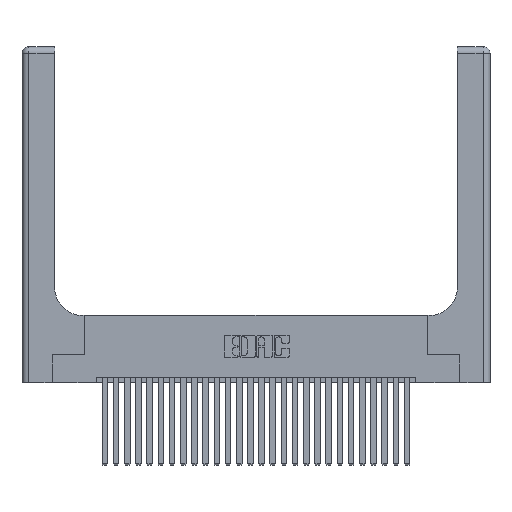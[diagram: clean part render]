
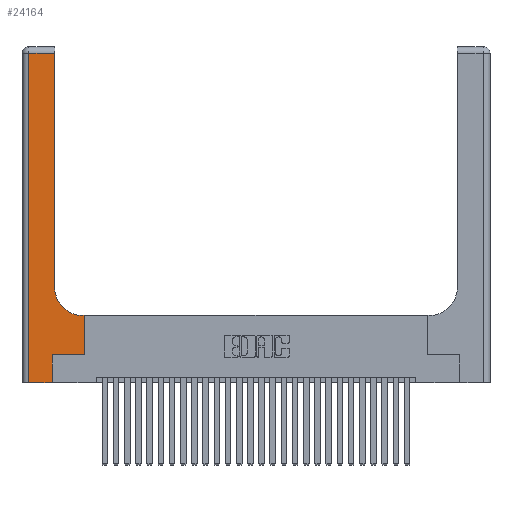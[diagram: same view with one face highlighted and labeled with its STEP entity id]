
A CAD part, top view. The second image highlights one B-rep face of the part: STEP entity #24164.
In plain terms, the highlighted planar face has unit normal (0, 0, 1).
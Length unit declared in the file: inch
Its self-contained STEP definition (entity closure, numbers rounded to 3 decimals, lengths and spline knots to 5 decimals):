
#298 = VERTEX_POINT ( 'NONE', #4008 ) ;
#327 = LINE ( 'NONE', #25647, #7044 ) ;
#1005 = VECTOR ( 'NONE', #8817, 39.37008 ) ;
#1125 = DIRECTION ( 'NONE',  ( 0., 0., -1. ) ) ;
#1407 = EDGE_CURVE ( 'NONE', #298, #4816, #18150, .T. ) ;
#1796 = ORIENTED_EDGE ( 'NONE', *, *, #18109, .T. ) ;
#2268 = EDGE_CURVE ( 'NONE', #15650, #21224, #3063, .T. ) ;
#2688 = VERTEX_POINT ( 'NONE', #15020 ) ;
#3062 = ORIENTED_EDGE ( 'NONE', *, *, #1407, .T. ) ;
#3063 = CIRCLE ( 'NONE', #17693, 0.25 ) ;
#3079 = DIRECTION ( 'NONE',  ( 1., 0., 0. ) ) ;
#3293 = CARTESIAN_POINT ( 'NONE',  ( 0.2915, 0.6, 0.37 ) ) ;
#3339 = CARTESIAN_POINT ( 'NONE',  ( 0.5585, 0.25, 0.37 ) ) ;
#3639 = CARTESIAN_POINT ( 'NONE',  ( 0.2915, 0.85, 0.37 ) ) ;
#4008 = CARTESIAN_POINT ( 'NONE',  ( 0.5585, 0.25, 0.37 ) ) ;
#4056 = CARTESIAN_POINT ( 'NONE',  ( 0.06, 3., 0.37 ) ) ;
#4513 = CARTESIAN_POINT ( 'NONE',  ( 0.5415, 0.85, 0.37 ) ) ;
#4816 = VERTEX_POINT ( 'NONE', #13047 ) ;
#5279 = LINE ( 'NONE', #3293, #16467 ) ;
#6472 = FACE_OUTER_BOUND ( 'NONE', #11373, .T. ) ;
#6727 = DIRECTION ( 'NONE',  ( 1., 0., 0. ) ) ;
#7044 = VECTOR ( 'NONE', #27852, 39.37008 ) ;
#7307 = LINE ( 'NONE', #4056, #13261 ) ;
#7729 = LINE ( 'NONE', #27632, #24783 ) ;
#7750 = CARTESIAN_POINT ( 'NONE',  ( 0.5415, 0.6, 0.37 ) ) ;
#7824 = DIRECTION ( 'NONE',  ( 0., 1., 0. ) ) ;
#8817 = DIRECTION ( 'NONE',  ( -1., 0., 0. ) ) ;
#9184 = EDGE_CURVE ( 'NONE', #19951, #298, #327, .T. ) ;
#9805 = VERTEX_POINT ( 'NONE', #23495 ) ;
#10004 = VECTOR ( 'NONE', #10326, 39.37008 ) ;
#10326 = DIRECTION ( 'NONE',  ( 0., 1., 0. ) ) ;
#10386 = ORIENTED_EDGE ( 'NONE', *, *, #2268, .T. ) ;
#10901 = EDGE_CURVE ( 'NONE', #9805, #2688, #12663, .T. ) ;
#11137 = CARTESIAN_POINT ( 'NONE',  ( 0.06, 2.94, 0.37 ) ) ;
#11282 = DIRECTION ( 'NONE',  ( 0., 1., 0. ) ) ;
#11373 = EDGE_LOOP ( 'NONE', ( #27351, #1796, #19914, #27807, #18780, #25518, #3062, #13620, #10386 ) ) ;
#11813 = DIRECTION ( 'NONE',  ( -1., 0., 0. ) ) ;
#12663 = LINE ( 'NONE', #20819, #23082 ) ;
#12683 = CARTESIAN_POINT ( 'NONE',  ( 0.2915, 2.94, 0.37 ) ) ;
#13047 = CARTESIAN_POINT ( 'NONE',  ( 0.5585, 0.6, 0.37 ) ) ;
#13261 = VECTOR ( 'NONE', #19632, 39.37008 ) ;
#13620 = ORIENTED_EDGE ( 'NONE', *, *, #27261, .T. ) ;
#15020 = CARTESIAN_POINT ( 'NONE',  ( 0.269, 0., 0.37 ) ) ;
#15332 = VERTEX_POINT ( 'NONE', #11137 ) ;
#15650 = VERTEX_POINT ( 'NONE', #7750 ) ;
#16467 = VECTOR ( 'NONE', #11813, 39.37008 ) ;
#16825 = DIRECTION ( 'NONE',  ( -1., 0., 0. ) ) ;
#17640 = EDGE_CURVE ( 'NONE', #21224, #24825, #7729, .T. ) ;
#17693 = AXIS2_PLACEMENT_3D ( 'NONE', #4513, #20079, #6727 ) ;
#17885 = CARTESIAN_POINT ( 'NONE',  ( 0.269, 0.25, 0.37 ) ) ;
#18109 = EDGE_CURVE ( 'NONE', #24825, #15332, #19564, .T. ) ;
#18150 = LINE ( 'NONE', #3339, #24010 ) ;
#18780 = ORIENTED_EDGE ( 'NONE', *, *, #23553, .T. ) ;
#19564 = LINE ( 'NONE', #19906, #1005 ) ;
#19632 = DIRECTION ( 'NONE',  ( 0., -1., 0. ) ) ;
#19906 = CARTESIAN_POINT ( 'NONE',  ( 0., 2.94, 0.37 ) ) ;
#19914 = ORIENTED_EDGE ( 'NONE', *, *, #28106, .T. ) ;
#19951 = VERTEX_POINT ( 'NONE', #17885 ) ;
#20079 = DIRECTION ( 'NONE',  ( 0., 0., -1. ) ) ;
#20819 = CARTESIAN_POINT ( 'NONE',  ( 0., 0., 0.37 ) ) ;
#21224 = VERTEX_POINT ( 'NONE', #3639 ) ;
#21373 = CARTESIAN_POINT ( 'NONE',  ( 0.269, 0., 0.37 ) ) ;
#21768 = AXIS2_PLACEMENT_3D ( 'NONE', #27799, #1125, #16825 ) ;
#21804 = LINE ( 'NONE', #21373, #10004 ) ;
#23082 = VECTOR ( 'NONE', #3079, 39.37008 ) ;
#23378 = PLANE ( 'NONE',  #21768 ) ;
#23495 = CARTESIAN_POINT ( 'NONE',  ( 0.06, 0., 0.37 ) ) ;
#23553 = EDGE_CURVE ( 'NONE', #2688, #19951, #21804, .T. ) ;
#24010 = VECTOR ( 'NONE', #7824, 39.37008 ) ;
#24164 = ADVANCED_FACE ( 'NONE', ( #6472 ), #23378, .F. ) ;
#24783 = VECTOR ( 'NONE', #11282, 39.37008 ) ;
#24825 = VERTEX_POINT ( 'NONE', #12683 ) ;
#25518 = ORIENTED_EDGE ( 'NONE', *, *, #9184, .T. ) ;
#25647 = CARTESIAN_POINT ( 'NONE',  ( 0.269, 0.25, 0.37 ) ) ;
#27261 = EDGE_CURVE ( 'NONE', #4816, #15650, #5279, .T. ) ;
#27351 = ORIENTED_EDGE ( 'NONE', *, *, #17640, .T. ) ;
#27632 = CARTESIAN_POINT ( 'NONE',  ( 0.2915, 3., 0.37 ) ) ;
#27799 = CARTESIAN_POINT ( 'NONE',  ( 0., 3., 0.37 ) ) ;
#27807 = ORIENTED_EDGE ( 'NONE', *, *, #10901, .T. ) ;
#27852 = DIRECTION ( 'NONE',  ( 1., 0., 0. ) ) ;
#28106 = EDGE_CURVE ( 'NONE', #15332, #9805, #7307, .T. ) ;
